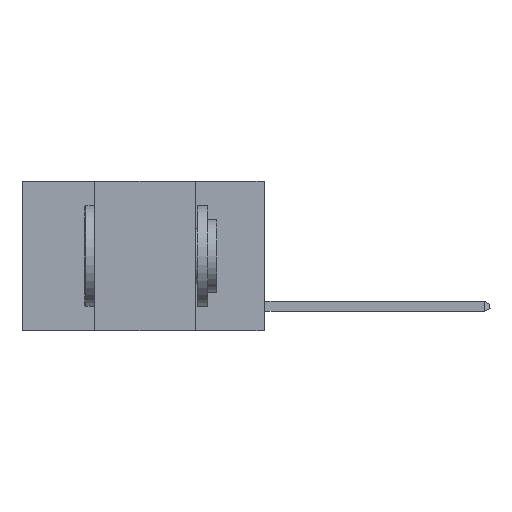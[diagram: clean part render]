
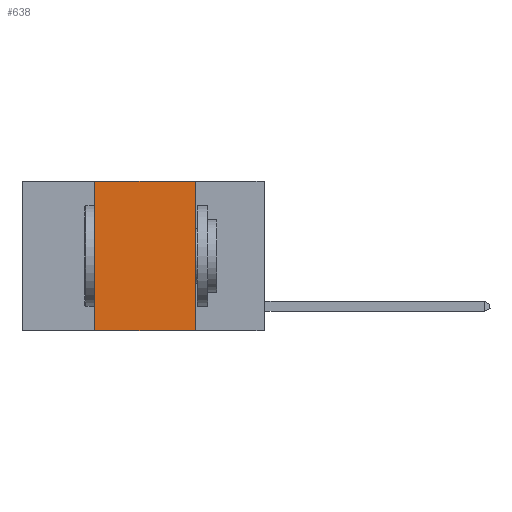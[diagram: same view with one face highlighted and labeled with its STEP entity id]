
A CAD part, left-side view. The second image highlights one B-rep face of the part: STEP entity #638.
In plain terms, the highlighted planar face has unit normal (-1, 0, 0).
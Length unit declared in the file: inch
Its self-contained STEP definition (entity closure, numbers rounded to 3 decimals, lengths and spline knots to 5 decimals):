
#178 = DIRECTION ( 'NONE',  ( 0., 0., 1. ) ) ;
#395 = DIRECTION ( 'NONE',  ( 0., 0., -1. ) ) ;
#638 = ADVANCED_FACE ( 'NONE', ( #1297 ), #5018, .F. ) ;
#1297 = FACE_OUTER_BOUND ( 'NONE', #7447, .T. ) ;
#1838 = VERTEX_POINT ( 'NONE', #10754 ) ;
#2218 = CARTESIAN_POINT ( 'NONE',  ( 0., 0.6, -0.37 ) ) ;
#2271 = VECTOR ( 'NONE', #9814, 39.37008 ) ;
#2339 = LINE ( 'NONE', #2218, #10353 ) ;
#2980 = VERTEX_POINT ( 'NONE', #11204 ) ;
#3182 = DIRECTION ( 'NONE',  ( 1., 0., 0. ) ) ;
#3243 = VECTOR ( 'NONE', #178, 39.37008 ) ;
#3566 = EDGE_CURVE ( 'NONE', #1838, #8776, #4991, .T. ) ;
#4991 = LINE ( 'NONE', #9676, #5929 ) ;
#5018 = PLANE ( 'NONE',  #8917 ) ;
#5855 = DIRECTION ( 'NONE',  ( 0., -1., 0. ) ) ;
#5929 = VECTOR ( 'NONE', #395, 39.37008 ) ;
#7196 = ORIENTED_EDGE ( 'NONE', *, *, #3566, .F. ) ;
#7206 = EDGE_CURVE ( 'NONE', #2980, #8776, #2339, .T. ) ;
#7447 = EDGE_LOOP ( 'NONE', ( #7196, #9070, #12041, #12115 ) ) ;
#7483 = CARTESIAN_POINT ( 'NONE',  ( 0., 0.42, 0. ) ) ;
#7907 = CARTESIAN_POINT ( 'NONE',  ( 0., 0.6, 0. ) ) ;
#8022 = CARTESIAN_POINT ( 'NONE',  ( 0., 0.6, 0. ) ) ;
#8155 = CARTESIAN_POINT ( 'NONE',  ( 0., 0.17, -0.37 ) ) ;
#8434 = EDGE_CURVE ( 'NONE', #2980, #11541, #12232, .T. ) ;
#8617 = EDGE_CURVE ( 'NONE', #11541, #1838, #10685, .T. ) ;
#8776 = VERTEX_POINT ( 'NONE', #8155 ) ;
#8917 = AXIS2_PLACEMENT_3D ( 'NONE', #7907, #3182, #10751 ) ;
#9070 = ORIENTED_EDGE ( 'NONE', *, *, #8617, .F. ) ;
#9642 = CARTESIAN_POINT ( 'NONE',  ( 0., 0.42, 0. ) ) ;
#9676 = CARTESIAN_POINT ( 'NONE',  ( 0., 0.17, 0. ) ) ;
#9814 = DIRECTION ( 'NONE',  ( 0., -1., 0. ) ) ;
#10353 = VECTOR ( 'NONE', #5855, 39.37008 ) ;
#10685 = LINE ( 'NONE', #8022, #2271 ) ;
#10751 = DIRECTION ( 'NONE',  ( 0., 0., -1. ) ) ;
#10754 = CARTESIAN_POINT ( 'NONE',  ( 0., 0.17, 0. ) ) ;
#11204 = CARTESIAN_POINT ( 'NONE',  ( 0., 0.42, -0.37 ) ) ;
#11541 = VERTEX_POINT ( 'NONE', #9642 ) ;
#12041 = ORIENTED_EDGE ( 'NONE', *, *, #8434, .F. ) ;
#12115 = ORIENTED_EDGE ( 'NONE', *, *, #7206, .T. ) ;
#12232 = LINE ( 'NONE', #7483, #3243 ) ;
